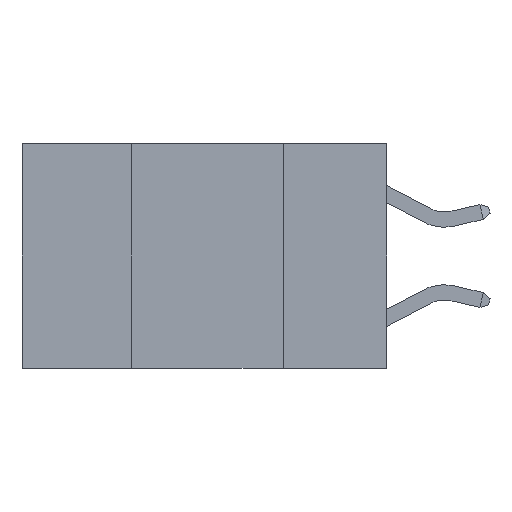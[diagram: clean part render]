
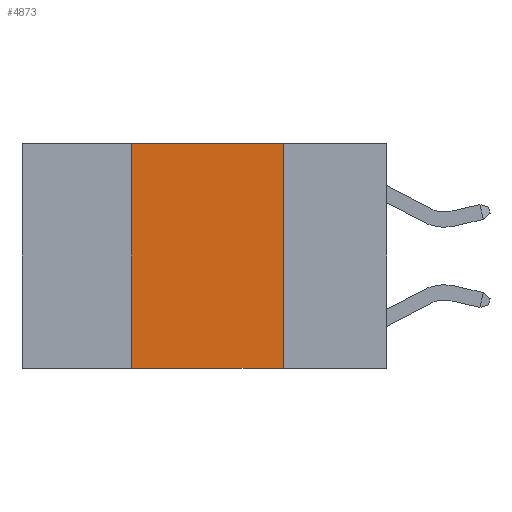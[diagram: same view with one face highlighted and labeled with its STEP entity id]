
A CAD part, left-side view. The second image highlights one B-rep face of the part: STEP entity #4873.
In plain terms, the highlighted planar face has unit normal (-1, 0, 0).
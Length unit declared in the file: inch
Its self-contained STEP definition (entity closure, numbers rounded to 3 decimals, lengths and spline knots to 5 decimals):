
#100 = CARTESIAN_POINT ( 'NONE',  ( 0., 0.6, -0.37 ) ) ;
#282 = ORIENTED_EDGE ( 'NONE', *, *, #1777, .F. ) ;
#928 = DIRECTION ( 'NONE',  ( 1., 0., 0. ) ) ;
#1221 = ORIENTED_EDGE ( 'NONE', *, *, #7815, .F. ) ;
#1241 = VERTEX_POINT ( 'NONE', #8388 ) ;
#1302 = VECTOR ( 'NONE', #10062, 39.37008 ) ;
#1434 = LINE ( 'NONE', #12093, #9279 ) ;
#1777 = EDGE_CURVE ( 'NONE', #8251, #1241, #1434, .T. ) ;
#3438 = DIRECTION ( 'NONE',  ( 0., -1., 0. ) ) ;
#3571 = CARTESIAN_POINT ( 'NONE',  ( 0., 0.42, -0.37 ) ) ;
#3904 = CARTESIAN_POINT ( 'NONE',  ( 0., 0.6, 0. ) ) ;
#4394 = LINE ( 'NONE', #8687, #5102 ) ;
#4703 = VERTEX_POINT ( 'NONE', #3571 ) ;
#4873 = ADVANCED_FACE ( 'NONE', ( #6228 ), #13707, .F. ) ;
#5102 = VECTOR ( 'NONE', #5384, 39.37008 ) ;
#5384 = DIRECTION ( 'NONE',  ( 0., 0., -1. ) ) ;
#5961 = AXIS2_PLACEMENT_3D ( 'NONE', #3904, #928, #9378 ) ;
#6005 = VECTOR ( 'NONE', #3438, 39.37008 ) ;
#6117 = VERTEX_POINT ( 'NONE', #8980 ) ;
#6228 = FACE_OUTER_BOUND ( 'NONE', #11209, .T. ) ;
#7815 = EDGE_CURVE ( 'NONE', #4703, #8251, #13758, .T. ) ;
#8121 = EDGE_CURVE ( 'NONE', #4703, #6117, #8705, .T. ) ;
#8251 = VERTEX_POINT ( 'NONE', #9894 ) ;
#8388 = CARTESIAN_POINT ( 'NONE',  ( 0., 0.17, 0. ) ) ;
#8687 = CARTESIAN_POINT ( 'NONE',  ( 0., 0.17, 0. ) ) ;
#8705 = LINE ( 'NONE', #100, #6005 ) ;
#8980 = CARTESIAN_POINT ( 'NONE',  ( 0., 0.17, -0.37 ) ) ;
#9279 = VECTOR ( 'NONE', #13197, 39.37008 ) ;
#9378 = DIRECTION ( 'NONE',  ( 0., 0., -1. ) ) ;
#9894 = CARTESIAN_POINT ( 'NONE',  ( 0., 0.42, 0. ) ) ;
#10062 = DIRECTION ( 'NONE',  ( 0., 0., 1. ) ) ;
#10957 = EDGE_CURVE ( 'NONE', #1241, #6117, #4394, .T. ) ;
#11209 = EDGE_LOOP ( 'NONE', ( #13411, #282, #1221, #12703 ) ) ;
#12093 = CARTESIAN_POINT ( 'NONE',  ( 0., 0.6, 0. ) ) ;
#12703 = ORIENTED_EDGE ( 'NONE', *, *, #8121, .T. ) ;
#12725 = CARTESIAN_POINT ( 'NONE',  ( 0., 0.42, 0. ) ) ;
#13197 = DIRECTION ( 'NONE',  ( 0., -1., 0. ) ) ;
#13411 = ORIENTED_EDGE ( 'NONE', *, *, #10957, .F. ) ;
#13707 = PLANE ( 'NONE',  #5961 ) ;
#13758 = LINE ( 'NONE', #12725, #1302 ) ;
